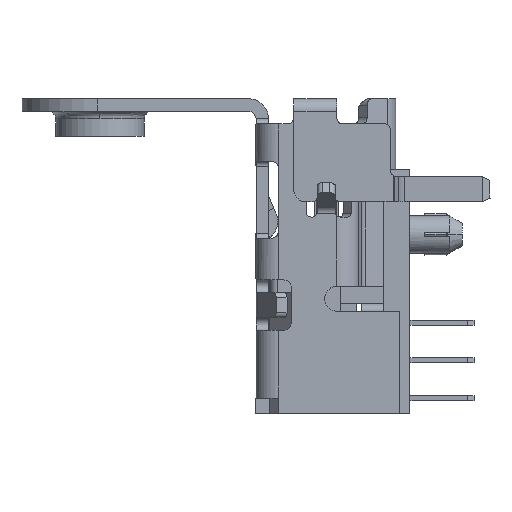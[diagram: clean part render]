
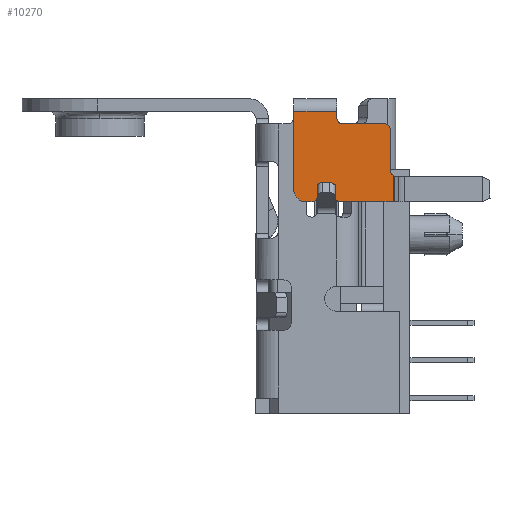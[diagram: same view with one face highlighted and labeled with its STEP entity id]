
A CAD part, left-side view. The second image highlights one B-rep face of the part: STEP entity #10270.
In plain terms, the highlighted face is planar.
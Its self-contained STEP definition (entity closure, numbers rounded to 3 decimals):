
#236 = ORIENTED_EDGE ( 'NONE', *, *, #68388, .T. ) ;
#355 = DIRECTION ( 'NONE',  ( 0., 0., 1. ) ) ;
#978 = CARTESIAN_POINT ( 'NONE',  ( 55.391, 58.475, -11.95 ) ) ;
#1343 = CIRCLE ( 'NONE', #48096, 0.25 ) ;
#1759 = AXIS2_PLACEMENT_3D ( 'NONE', #26790, #27149, #42144 ) ;
#1832 = ORIENTED_EDGE ( 'NONE', *, *, #39693, .T. ) ;
#1912 = AXIS2_PLACEMENT_3D ( 'NONE', #24295, #3019, #2343 ) ;
#2343 = DIRECTION ( 'NONE',  ( 0., 0., 1. ) ) ;
#2472 = CARTESIAN_POINT ( 'NONE',  ( 55.391, 60.121, -11.95 ) ) ;
#2474 = DIRECTION ( 'NONE',  ( 0., 0., 1. ) ) ;
#2744 = VERTEX_POINT ( 'NONE', #44087 ) ;
#2913 = LINE ( 'NONE', #66052, #17195 ) ;
#3019 = DIRECTION ( 'NONE',  ( 1., 0., 0. ) ) ;
#3222 = VERTEX_POINT ( 'NONE', #2472 ) ;
#3659 = LINE ( 'NONE', #24927, #38132 ) ;
#4093 = CARTESIAN_POINT ( 'NONE',  ( 55.391, 57.975, -10.1 ) ) ;
#4342 = CARTESIAN_POINT ( 'NONE',  ( 55.391, 61.145, -9.05 ) ) ;
#4474 = CARTESIAN_POINT ( 'NONE',  ( 55.391, 60.371, -12.2 ) ) ;
#4756 = DIRECTION ( 'NONE',  ( 0., 1., 0. ) ) ;
#5646 = ORIENTED_EDGE ( 'NONE', *, *, #12316, .T. ) ;
#5711 = ORIENTED_EDGE ( 'NONE', *, *, #42529, .F. ) ;
#6128 = ORIENTED_EDGE ( 'NONE', *, *, #60483, .T. ) ;
#6296 = CARTESIAN_POINT ( 'NONE',  ( 55.391, 61.345, -8.85 ) ) ;
#6441 = ORIENTED_EDGE ( 'NONE', *, *, #33829, .T. ) ;
#7458 = DIRECTION ( 'NONE',  ( 0., -1., 0. ) ) ;
#7755 = CARTESIAN_POINT ( 'NONE',  ( 55.391, 61.145, -10.65 ) ) ;
#8191 = CARTESIAN_POINT ( 'NONE',  ( 55.391, 60.371, -12.45 ) ) ;
#8526 = DIRECTION ( 'NONE',  ( 0., 0., -1. ) ) ;
#9298 = CARTESIAN_POINT ( 'NONE',  ( 55.391, 60.225, -9.05 ) ) ;
#10270 = ADVANCED_FACE ( 'NONE', ( #54681 ), #13478, .T. ) ;
#11445 = CARTESIAN_POINT ( 'NONE',  ( 55.391, 60.425, -9.56 ) ) ;
#12316 = EDGE_CURVE ( 'NONE', #13955, #24832, #20203, .T. ) ;
#13313 = ORIENTED_EDGE ( 'NONE', *, *, #44470, .F. ) ;
#13478 = PLANE ( 'NONE',  #1912 ) ;
#13610 = LINE ( 'NONE', #55155, #44043 ) ;
#13742 = CARTESIAN_POINT ( 'NONE',  ( 55.391, 59.298, -11.95 ) ) ;
#13955 = VERTEX_POINT ( 'NONE', #4342 ) ;
#14265 = CARTESIAN_POINT ( 'NONE',  ( 55.391, 60.121, -12.2 ) ) ;
#14376 = DIRECTION ( 'NONE',  ( 0., 0., -1. ) ) ;
#14384 = CARTESIAN_POINT ( 'NONE',  ( 55.391, 58.225, -10.1 ) ) ;
#14886 = DIRECTION ( 'NONE',  ( 0., 0., -1. ) ) ;
#15467 = VERTEX_POINT ( 'NONE', #18014 ) ;
#16022 = CARTESIAN_POINT ( 'NONE',  ( 55.391, 60.425, -10.65 ) ) ;
#16478 = AXIS2_PLACEMENT_3D ( 'NONE', #68081, #40582, #14376 ) ;
#16527 = VECTOR ( 'NONE', #41487, 1000. ) ;
#16534 = CARTESIAN_POINT ( 'NONE',  ( 55.391, 60.425, -9.05 ) ) ;
#17195 = VECTOR ( 'NONE', #7458, 1000. ) ;
#18014 = CARTESIAN_POINT ( 'NONE',  ( 55.391, 61.575, -8.85 ) ) ;
#18464 = CARTESIAN_POINT ( 'NONE',  ( 55.391, 58.225, -10.65 ) ) ;
#18664 = VERTEX_POINT ( 'NONE', #46124 ) ;
#19096 = EDGE_CURVE ( 'NONE', #49715, #37852, #56092, .T. ) ;
#19953 = VERTEX_POINT ( 'NONE', #6296 ) ;
#20203 = LINE ( 'NONE', #7755, #16527 ) ;
#20347 = ORIENTED_EDGE ( 'NONE', *, *, #56429, .T. ) ;
#20455 = AXIS2_PLACEMENT_3D ( 'NONE', #9298, #61271, #34794 ) ;
#20798 = CARTESIAN_POINT ( 'NONE',  ( 55.391, 60.1, -12.45 ) ) ;
#20933 = ORIENTED_EDGE ( 'NONE', *, *, #51938, .T. ) ;
#21791 = EDGE_CURVE ( 'NONE', #28556, #60447, #68562, .T. ) ;
#22165 = VERTEX_POINT ( 'NONE', #48193 ) ;
#22499 = CARTESIAN_POINT ( 'NONE',  ( 55.391, 62.154, -9.56 ) ) ;
#22926 = VECTOR ( 'NONE', #23689, 1000. ) ;
#23689 = DIRECTION ( 'NONE',  ( 0., 0., -1. ) ) ;
#24295 = CARTESIAN_POINT ( 'NONE',  ( 55.391, 62.154, -12.522 ) ) ;
#24832 = VERTEX_POINT ( 'NONE', #55795 ) ;
#24927 = CARTESIAN_POINT ( 'NONE',  ( 55.391, 58.125, -10.65 ) ) ;
#25031 = DIRECTION ( 'NONE',  ( 1., 0., 0. ) ) ;
#25219 = VECTOR ( 'NONE', #52005, 1000. ) ;
#26406 = CARTESIAN_POINT ( 'NONE',  ( 55.391, 61.575, -9.35 ) ) ;
#26595 = AXIS2_PLACEMENT_3D ( 'NONE', #4093, #56417, #52575 ) ;
#26739 = EDGE_CURVE ( 'NONE', #67172, #28556, #65759, .T. ) ;
#26790 = CARTESIAN_POINT ( 'NONE',  ( 55.391, 61.345, -9.05 ) ) ;
#26846 = VECTOR ( 'NONE', #50740, 1000. ) ;
#26863 = EDGE_CURVE ( 'NONE', #22165, #18664, #3659, .T. ) ;
#27149 = DIRECTION ( 'NONE',  ( 1., 0., 0. ) ) ;
#27405 = VERTEX_POINT ( 'NONE', #29901 ) ;
#27416 = VECTOR ( 'NONE', #61432, 1000. ) ;
#28556 = VERTEX_POINT ( 'NONE', #8191 ) ;
#29901 = CARTESIAN_POINT ( 'NONE',  ( 55.391, 58.225, -11.7 ) ) ;
#31364 = ORIENTED_EDGE ( 'NONE', *, *, #26863, .T. ) ;
#33489 = LINE ( 'NONE', #18464, #22926 ) ;
#33829 = EDGE_CURVE ( 'NONE', #48575, #27405, #33489, .T. ) ;
#34780 = ORIENTED_EDGE ( 'NONE', *, *, #19096, .T. ) ;
#34794 = DIRECTION ( 'NONE',  ( 0., 0., -1. ) ) ;
#35228 = DIRECTION ( 'NONE',  ( 1., 0., 0. ) ) ;
#36595 = DIRECTION ( 'NONE',  ( 0., 0., 1. ) ) ;
#36638 = CIRCLE ( 'NONE', #26595, 0.25 ) ;
#36900 = EDGE_CURVE ( 'NONE', #27405, #53116, #57713, .T. ) ;
#37852 = VERTEX_POINT ( 'NONE', #61147 ) ;
#38132 = VECTOR ( 'NONE', #46228, 1000. ) ;
#39693 = EDGE_CURVE ( 'NONE', #18664, #48575, #36638, .T. ) ;
#40301 = CARTESIAN_POINT ( 'NONE',  ( 55.391, 60.371, -12.325 ) ) ;
#40582 = DIRECTION ( 'NONE',  ( 1., 0., 0. ) ) ;
#41487 = DIRECTION ( 'NONE',  ( 0., 0., -1. ) ) ;
#41890 = LINE ( 'NONE', #52692, #25219 ) ;
#42144 = DIRECTION ( 'NONE',  ( 0., 0., -1. ) ) ;
#42529 = EDGE_CURVE ( 'NONE', #3222, #53116, #45863, .T. ) ;
#43709 = VECTOR ( 'NONE', #8526, 1000. ) ;
#44043 = VECTOR ( 'NONE', #2474, 1000. ) ;
#44087 = CARTESIAN_POINT ( 'NONE',  ( 55.391, 62.075, -9.35 ) ) ;
#44133 = LINE ( 'NONE', #22499, #27416 ) ;
#44470 = EDGE_CURVE ( 'NONE', #67172, #3222, #1343, .T. ) ;
#45863 = LINE ( 'NONE', #13742, #26846 ) ;
#46124 = CARTESIAN_POINT ( 'NONE',  ( 55.391, 58.125, -9.9 ) ) ;
#46228 = DIRECTION ( 'NONE',  ( 0., 0., -1. ) ) ;
#47700 = EDGE_CURVE ( 'NONE', #2744, #15467, #50486, .T. ) ;
#48096 = AXIS2_PLACEMENT_3D ( 'NONE', #14265, #35228, #36595 ) ;
#48176 = VECTOR ( 'NONE', #355, 1000. ) ;
#48193 = CARTESIAN_POINT ( 'NONE',  ( 55.391, 58.125, -8.85 ) ) ;
#48575 = VERTEX_POINT ( 'NONE', #14384 ) ;
#49522 = EDGE_CURVE ( 'NONE', #37852, #22165, #2913, .T. ) ;
#49715 = VERTEX_POINT ( 'NONE', #16534 ) ;
#50486 = CIRCLE ( 'NONE', #56038, 0.5 ) ;
#50740 = DIRECTION ( 'NONE',  ( 0., -1., 0. ) ) ;
#51287 = ORIENTED_EDGE ( 'NONE', *, *, #49522, .T. ) ;
#51938 = EDGE_CURVE ( 'NONE', #19953, #13955, #64056, .T. ) ;
#52005 = DIRECTION ( 'NONE',  ( 0., -1., 0. ) ) ;
#52517 = EDGE_CURVE ( 'NONE', #24832, #62807, #44133, .T. ) ;
#52575 = DIRECTION ( 'NONE',  ( 0., 0., 1. ) ) ;
#52692 = CARTESIAN_POINT ( 'NONE',  ( 55.391, 60.1, -8.85 ) ) ;
#53116 = VERTEX_POINT ( 'NONE', #978 ) ;
#54681 = FACE_OUTER_BOUND ( 'NONE', #55262, .T. ) ;
#55155 = CARTESIAN_POINT ( 'NONE',  ( 55.391, 62.075, -10.65 ) ) ;
#55262 = EDGE_LOOP ( 'NONE', ( #64948, #236, #34780, #51287, #31364, #1832, #6441, #57956, #5711, #13313, #66181, #57041, #20347, #67685, #6128, #20933, #5646 ) ) ;
#55795 = CARTESIAN_POINT ( 'NONE',  ( 55.391, 61.145, -9.56 ) ) ;
#56038 = AXIS2_PLACEMENT_3D ( 'NONE', #26406, #25031, #14886 ) ;
#56092 = CIRCLE ( 'NONE', #20455, 0.2 ) ;
#56417 = DIRECTION ( 'NONE',  ( -1., 0., 0. ) ) ;
#56429 = EDGE_CURVE ( 'NONE', #60447, #2744, #13610, .T. ) ;
#57041 = ORIENTED_EDGE ( 'NONE', *, *, #21791, .T. ) ;
#57713 = CIRCLE ( 'NONE', #16478, 0.25 ) ;
#57956 = ORIENTED_EDGE ( 'NONE', *, *, #36900, .T. ) ;
#58233 = LINE ( 'NONE', #16022, #48176 ) ;
#60447 = VERTEX_POINT ( 'NONE', #67688 ) ;
#60483 = EDGE_CURVE ( 'NONE', #15467, #19953, #41890, .T. ) ;
#61147 = CARTESIAN_POINT ( 'NONE',  ( 55.391, 60.225, -8.85 ) ) ;
#61271 = DIRECTION ( 'NONE',  ( 1., 0., 0. ) ) ;
#61432 = DIRECTION ( 'NONE',  ( 0., -1., 0. ) ) ;
#62807 = VERTEX_POINT ( 'NONE', #11445 ) ;
#64056 = CIRCLE ( 'NONE', #1759, 0.2 ) ;
#64948 = ORIENTED_EDGE ( 'NONE', *, *, #52517, .T. ) ;
#65759 = LINE ( 'NONE', #40301, #43709 ) ;
#66052 = CARTESIAN_POINT ( 'NONE',  ( 55.391, 60.1, -8.85 ) ) ;
#66181 = ORIENTED_EDGE ( 'NONE', *, *, #26739, .T. ) ;
#67172 = VERTEX_POINT ( 'NONE', #4474 ) ;
#67685 = ORIENTED_EDGE ( 'NONE', *, *, #47700, .T. ) ;
#67688 = CARTESIAN_POINT ( 'NONE',  ( 55.391, 62.075, -12.45 ) ) ;
#68081 = CARTESIAN_POINT ( 'NONE',  ( 55.391, 58.475, -11.7 ) ) ;
#68388 = EDGE_CURVE ( 'NONE', #62807, #49715, #58233, .T. ) ;
#68562 = LINE ( 'NONE', #20798, #68864 ) ;
#68864 = VECTOR ( 'NONE', #4756, 1000. ) ;
